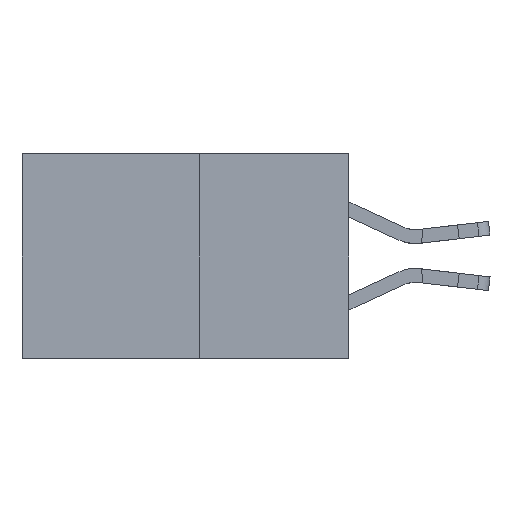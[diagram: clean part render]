
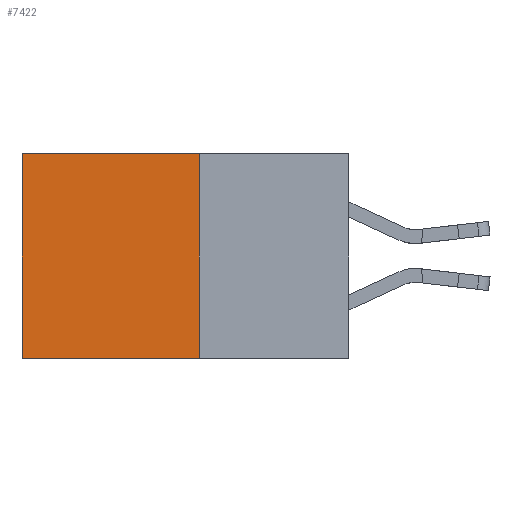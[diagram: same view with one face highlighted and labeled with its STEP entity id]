
A CAD part, left-side view. The second image highlights one B-rep face of the part: STEP entity #7422.
In plain terms, the highlighted planar face has unit normal (-1, 0, 0).
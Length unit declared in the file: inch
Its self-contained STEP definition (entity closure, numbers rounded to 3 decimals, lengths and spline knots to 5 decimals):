
#433 = ORIENTED_EDGE ( 'NONE', *, *, #26734, .T. ) ;
#441 = VECTOR ( 'NONE', #22868, 39.37008 ) ;
#608 = VECTOR ( 'NONE', #21408, 39.37008 ) ;
#658 = DIRECTION ( 'NONE',  ( 0., 0., -1. ) ) ;
#3365 = LINE ( 'NONE', #11641, #8491 ) ;
#3914 = VERTEX_POINT ( 'NONE', #12668 ) ;
#4578 = EDGE_CURVE ( 'NONE', #3914, #26208, #18884, .T. ) ;
#5265 = CARTESIAN_POINT ( 'NONE',  ( 0.277, 0.27, -0.37 ) ) ;
#5459 = EDGE_LOOP ( 'NONE', ( #22330, #9945, #24343, #433 ) ) ;
#6303 = VERTEX_POINT ( 'NONE', #16755 ) ;
#7422 = ADVANCED_FACE ( 'NONE', ( #25536 ), #12409, .F. ) ;
#8491 = VECTOR ( 'NONE', #658, 39.37008 ) ;
#8878 = VERTEX_POINT ( 'NONE', #23675 ) ;
#9244 = DIRECTION ( 'NONE',  ( 0., 1., 0. ) ) ;
#9945 = ORIENTED_EDGE ( 'NONE', *, *, #4578, .F. ) ;
#9961 = VECTOR ( 'NONE', #9244, 39.37008 ) ;
#9987 = EDGE_CURVE ( 'NONE', #8878, #3914, #24550, .T. ) ;
#11641 = CARTESIAN_POINT ( 'NONE',  ( 0.277, 0.59, -0.37 ) ) ;
#12314 = DIRECTION ( 'NONE',  ( 0., 0., -1. ) ) ;
#12376 = DIRECTION ( 'NONE',  ( 1., 0., 0. ) ) ;
#12400 = CARTESIAN_POINT ( 'NONE',  ( 0.277, 0.27, -0.37 ) ) ;
#12409 = PLANE ( 'NONE',  #24226 ) ;
#12668 = CARTESIAN_POINT ( 'NONE',  ( 0.277, 0.27, -0.37 ) ) ;
#14410 = EDGE_CURVE ( 'NONE', #6303, #26208, #3365, .T. ) ;
#16755 = CARTESIAN_POINT ( 'NONE',  ( 0.277, 0.59, 0. ) ) ;
#18884 = LINE ( 'NONE', #21555, #608 ) ;
#21408 = DIRECTION ( 'NONE',  ( 0., 1., 0. ) ) ;
#21555 = CARTESIAN_POINT ( 'NONE',  ( 0.277, 0.27, -0.37 ) ) ;
#22330 = ORIENTED_EDGE ( 'NONE', *, *, #14410, .T. ) ;
#22441 = CARTESIAN_POINT ( 'NONE',  ( 0.277, 0.27, 0. ) ) ;
#22868 = DIRECTION ( 'NONE',  ( 0., 0., -1. ) ) ;
#23675 = CARTESIAN_POINT ( 'NONE',  ( 0.277, 0.27, 0. ) ) ;
#24226 = AXIS2_PLACEMENT_3D ( 'NONE', #12400, #12376, #12314 ) ;
#24343 = ORIENTED_EDGE ( 'NONE', *, *, #9987, .F. ) ;
#24550 = LINE ( 'NONE', #5265, #441 ) ;
#25124 = CARTESIAN_POINT ( 'NONE',  ( 0.277, 0.59, -0.37 ) ) ;
#25536 = FACE_OUTER_BOUND ( 'NONE', #5459, .T. ) ;
#26208 = VERTEX_POINT ( 'NONE', #25124 ) ;
#26734 = EDGE_CURVE ( 'NONE', #8878, #6303, #28111, .T. ) ;
#28111 = LINE ( 'NONE', #22441, #9961 ) ;
